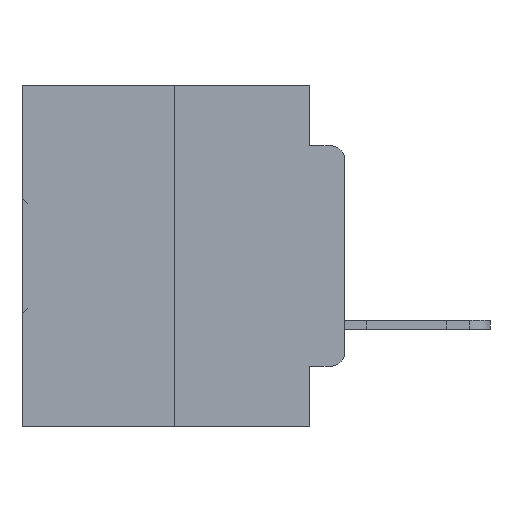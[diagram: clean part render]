
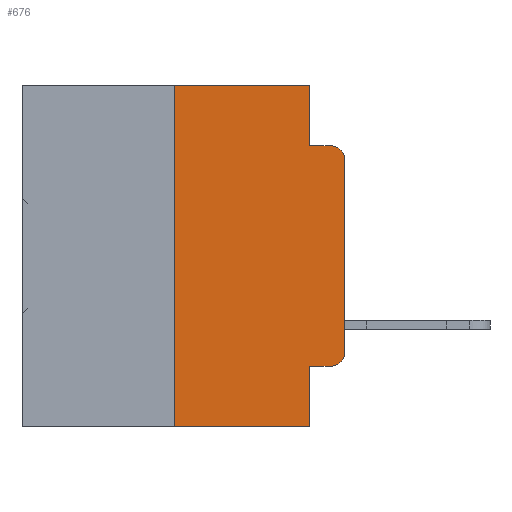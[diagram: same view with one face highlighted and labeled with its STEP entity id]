
A CAD part, left-side view. The second image highlights one B-rep face of the part: STEP entity #676.
In plain terms, the highlighted planar face has unit normal (-1, 0, 0).
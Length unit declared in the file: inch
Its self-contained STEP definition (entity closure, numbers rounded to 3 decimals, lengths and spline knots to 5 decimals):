
#65 = DIRECTION ( 'NONE',  ( 0., 0., 1. ) ) ;
#93 = CARTESIAN_POINT ( 'NONE',  ( 0., 0.051, -0.0885 ) ) ;
#676 = ADVANCED_FACE ( 'NONE', ( #22693 ), #21173, .F. ) ;
#1297 = LINE ( 'NONE', #12187, #8049 ) ;
#1437 = DIRECTION ( 'NONE',  ( 0., 0., -1. ) ) ;
#1492 = CARTESIAN_POINT ( 'NONE',  ( 0., 0.25, 0. ) ) ;
#1829 = LINE ( 'NONE', #15386, #8530 ) ;
#2165 = VECTOR ( 'NONE', #65, 39.37008 ) ;
#2638 = VECTOR ( 'NONE', #29113, 39.37008 ) ;
#2872 = CARTESIAN_POINT ( 'NONE',  ( 0., 0.02, -0.4115 ) ) ;
#3007 = CARTESIAN_POINT ( 'NONE',  ( 0., 0.25, 0. ) ) ;
#3066 = ORIENTED_EDGE ( 'NONE', *, *, #10043, .F. ) ;
#3111 = VERTEX_POINT ( 'NONE', #2872 ) ;
#3423 = CIRCLE ( 'NONE', #7850, 0.02 ) ;
#3600 = CARTESIAN_POINT ( 'NONE',  ( 0., 0.473, 0. ) ) ;
#3634 = EDGE_LOOP ( 'NONE', ( #21634, #4768, #14549, #12689, #3066, #13662, #28673, #18277, #22547, #4396 ) ) ;
#4373 = VERTEX_POINT ( 'NONE', #32197 ) ;
#4396 = ORIENTED_EDGE ( 'NONE', *, *, #17869, .T. ) ;
#4768 = ORIENTED_EDGE ( 'NONE', *, *, #13679, .T. ) ;
#4949 = CARTESIAN_POINT ( 'NONE',  ( 0., 0.02, -0.0885 ) ) ;
#5306 = CARTESIAN_POINT ( 'NONE',  ( 0., 0.473, -0.5 ) ) ;
#6027 = DIRECTION ( 'NONE',  ( 0., 0., -1. ) ) ;
#6185 = EDGE_CURVE ( 'NONE', #29050, #18974, #1297, .T. ) ;
#6489 = VERTEX_POINT ( 'NONE', #1492 ) ;
#6540 = VECTOR ( 'NONE', #12373, 39.37008 ) ;
#6548 = AXIS2_PLACEMENT_3D ( 'NONE', #3600, #6621, #6027 ) ;
#6621 = DIRECTION ( 'NONE',  ( 1., 0., 0. ) ) ;
#6639 = CARTESIAN_POINT ( 'NONE',  ( 0., 0.051, -0.5 ) ) ;
#6985 = VERTEX_POINT ( 'NONE', #6639 ) ;
#7850 = AXIS2_PLACEMENT_3D ( 'NONE', #16300, #16192, #16164 ) ;
#8049 = VECTOR ( 'NONE', #12747, 39.37008 ) ;
#8154 = DIRECTION ( 'NONE',  ( 0., -1., 0. ) ) ;
#8530 = VECTOR ( 'NONE', #1437, 39.37008 ) ;
#9630 = CARTESIAN_POINT ( 'NONE',  ( 0., 0., -0.1085 ) ) ;
#10043 = EDGE_CURVE ( 'NONE', #6489, #4373, #11723, .T. ) ;
#10444 = CARTESIAN_POINT ( 'NONE',  ( 0., 0., 0. ) ) ;
#10661 = LINE ( 'NONE', #3007, #2165 ) ;
#10951 = LINE ( 'NONE', #5306, #17165 ) ;
#11630 = CARTESIAN_POINT ( 'NONE',  ( 0., 0.473, 0. ) ) ;
#11723 = LINE ( 'NONE', #11630, #29609 ) ;
#11955 = CARTESIAN_POINT ( 'NONE',  ( 0., 0.25, -0.5 ) ) ;
#12187 = CARTESIAN_POINT ( 'NONE',  ( 0., 0.051, -0.0885 ) ) ;
#12373 = DIRECTION ( 'NONE',  ( 0., 0., 1. ) ) ;
#12689 = ORIENTED_EDGE ( 'NONE', *, *, #33669, .F. ) ;
#12747 = DIRECTION ( 'NONE',  ( 0., -1., 0. ) ) ;
#13609 = VERTEX_POINT ( 'NONE', #18178 ) ;
#13662 = ORIENTED_EDGE ( 'NONE', *, *, #32049, .F. ) ;
#13679 = EDGE_CURVE ( 'NONE', #17387, #18974, #3423, .T. ) ;
#14549 = ORIENTED_EDGE ( 'NONE', *, *, #6185, .F. ) ;
#14760 = LINE ( 'NONE', #10444, #6540 ) ;
#15386 = CARTESIAN_POINT ( 'NONE',  ( 0., 0.051, 0. ) ) ;
#15410 = EDGE_CURVE ( 'NONE', #13609, #17387, #14760, .T. ) ;
#15443 = DIRECTION ( 'NONE',  ( 0., -1., 0. ) ) ;
#16164 = DIRECTION ( 'NONE',  ( 0., 0., -1. ) ) ;
#16192 = DIRECTION ( 'NONE',  ( -1., 0., 0. ) ) ;
#16300 = CARTESIAN_POINT ( 'NONE',  ( 0., 0.02, -0.1085 ) ) ;
#16467 = LINE ( 'NONE', #28340, #2638 ) ;
#17165 = VECTOR ( 'NONE', #8154, 39.37008 ) ;
#17269 = CARTESIAN_POINT ( 'NONE',  ( 0., 0.051, 0. ) ) ;
#17387 = VERTEX_POINT ( 'NONE', #9630 ) ;
#17869 = EDGE_CURVE ( 'NONE', #3111, #13609, #34956, .T. ) ;
#18178 = CARTESIAN_POINT ( 'NONE',  ( 0., 0., -0.3915 ) ) ;
#18277 = ORIENTED_EDGE ( 'NONE', *, *, #30346, .F. ) ;
#18974 = VERTEX_POINT ( 'NONE', #4949 ) ;
#19686 = EDGE_CURVE ( 'NONE', #31255, #3111, #16467, .T. ) ;
#19749 = DIRECTION ( 'NONE',  ( 0., 0., -1. ) ) ;
#19976 = DIRECTION ( 'NONE',  ( -1., 0., 0. ) ) ;
#19982 = CARTESIAN_POINT ( 'NONE',  ( 0., 0.02, -0.3915 ) ) ;
#20037 = DIRECTION ( 'NONE',  ( 0., 0., -1. ) ) ;
#21173 = PLANE ( 'NONE',  #6548 ) ;
#21634 = ORIENTED_EDGE ( 'NONE', *, *, #15410, .T. ) ;
#22547 = ORIENTED_EDGE ( 'NONE', *, *, #19686, .T. ) ;
#22693 = FACE_OUTER_BOUND ( 'NONE', #3634, .T. ) ;
#26722 = EDGE_CURVE ( 'NONE', #30033, #6985, #10951, .T. ) ;
#28066 = CARTESIAN_POINT ( 'NONE',  ( 0., 0.051, -0.4115 ) ) ;
#28340 = CARTESIAN_POINT ( 'NONE',  ( 0., 0.051, -0.4115 ) ) ;
#28673 = ORIENTED_EDGE ( 'NONE', *, *, #26722, .T. ) ;
#29050 = VERTEX_POINT ( 'NONE', #93 ) ;
#29113 = DIRECTION ( 'NONE',  ( 0., -1., 0. ) ) ;
#29609 = VECTOR ( 'NONE', #15443, 39.37008 ) ;
#30033 = VERTEX_POINT ( 'NONE', #11955 ) ;
#30346 = EDGE_CURVE ( 'NONE', #31255, #6985, #1829, .T. ) ;
#31255 = VERTEX_POINT ( 'NONE', #28066 ) ;
#32049 = EDGE_CURVE ( 'NONE', #30033, #6489, #10661, .T. ) ;
#32197 = CARTESIAN_POINT ( 'NONE',  ( 0., 0.051, 0. ) ) ;
#33669 = EDGE_CURVE ( 'NONE', #4373, #29050, #35010, .T. ) ;
#33926 = AXIS2_PLACEMENT_3D ( 'NONE', #19982, #19976, #19749 ) ;
#34255 = VECTOR ( 'NONE', #20037, 39.37008 ) ;
#34956 = CIRCLE ( 'NONE', #33926, 0.02 ) ;
#35010 = LINE ( 'NONE', #17269, #34255 ) ;
